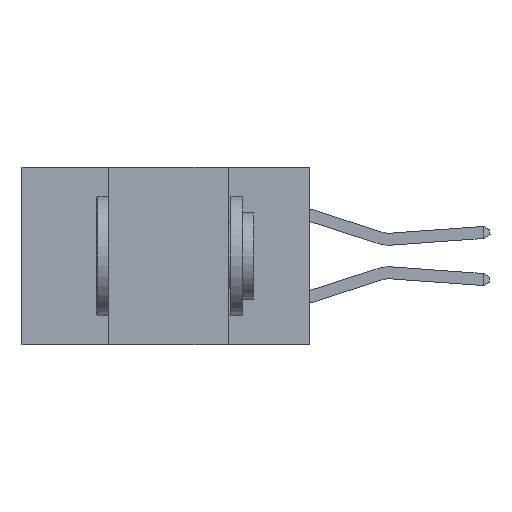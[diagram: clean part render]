
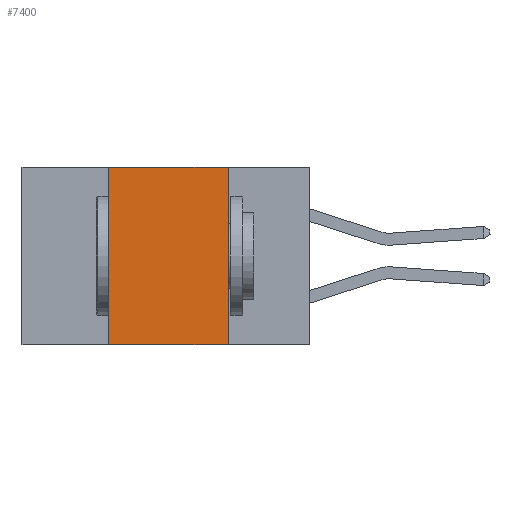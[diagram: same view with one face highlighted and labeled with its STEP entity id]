
A CAD part, left-side view. The second image highlights one B-rep face of the part: STEP entity #7400.
In plain terms, the highlighted planar face has unit normal (-1, 0, 0).
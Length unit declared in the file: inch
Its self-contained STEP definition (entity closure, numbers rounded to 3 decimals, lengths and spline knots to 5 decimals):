
#348 = DIRECTION ( 'NONE',  ( 1., 0., 0. ) ) ;
#670 = DIRECTION ( 'NONE',  ( 0., -1., 0. ) ) ;
#845 = CARTESIAN_POINT ( 'NONE',  ( 0., 0.6, 0. ) ) ;
#970 = VERTEX_POINT ( 'NONE', #16342 ) ;
#4624 = LINE ( 'NONE', #15076, #7123 ) ;
#5037 = EDGE_CURVE ( 'NONE', #16337, #5804, #14171, .T. ) ;
#5453 = ORIENTED_EDGE ( 'NONE', *, *, #18565, .T. ) ;
#5486 = VECTOR ( 'NONE', #18197, 39.37008 ) ;
#5804 = VERTEX_POINT ( 'NONE', #15506 ) ;
#5982 = ORIENTED_EDGE ( 'NONE', *, *, #14005, .F. ) ;
#6254 = EDGE_LOOP ( 'NONE', ( #5982, #7475, #9802, #5453 ) ) ;
#6794 = LINE ( 'NONE', #16508, #7512 ) ;
#7123 = VECTOR ( 'NONE', #11762, 39.37008 ) ;
#7400 = ADVANCED_FACE ( 'NONE', ( #11366 ), #9693, .F. ) ;
#7475 = ORIENTED_EDGE ( 'NONE', *, *, #5037, .F. ) ;
#7512 = VECTOR ( 'NONE', #670, 39.37008 ) ;
#7846 = AXIS2_PLACEMENT_3D ( 'NONE', #16038, #348, #16376 ) ;
#7856 = CARTESIAN_POINT ( 'NONE',  ( 0., 0.42, -0.37 ) ) ;
#8217 = DIRECTION ( 'NONE',  ( 0., 0., -1. ) ) ;
#8296 = EDGE_CURVE ( 'NONE', #15723, #16337, #4624, .T. ) ;
#9693 = PLANE ( 'NONE',  #7846 ) ;
#9802 = ORIENTED_EDGE ( 'NONE', *, *, #8296, .F. ) ;
#10439 = CARTESIAN_POINT ( 'NONE',  ( 0., 0.42, 0. ) ) ;
#11366 = FACE_OUTER_BOUND ( 'NONE', #6254, .T. ) ;
#11762 = DIRECTION ( 'NONE',  ( 0., 0., 1. ) ) ;
#12466 = LINE ( 'NONE', #17686, #19865 ) ;
#14005 = EDGE_CURVE ( 'NONE', #5804, #970, #12466, .T. ) ;
#14171 = LINE ( 'NONE', #845, #5486 ) ;
#15076 = CARTESIAN_POINT ( 'NONE',  ( 0., 0.42, 0. ) ) ;
#15506 = CARTESIAN_POINT ( 'NONE',  ( 0., 0.17, 0. ) ) ;
#15723 = VERTEX_POINT ( 'NONE', #7856 ) ;
#16038 = CARTESIAN_POINT ( 'NONE',  ( 0., 0.6, 0. ) ) ;
#16337 = VERTEX_POINT ( 'NONE', #10439 ) ;
#16342 = CARTESIAN_POINT ( 'NONE',  ( 0., 0.17, -0.37 ) ) ;
#16376 = DIRECTION ( 'NONE',  ( 0., 0., -1. ) ) ;
#16508 = CARTESIAN_POINT ( 'NONE',  ( 0., 0.6, -0.37 ) ) ;
#17686 = CARTESIAN_POINT ( 'NONE',  ( 0., 0.17, 0. ) ) ;
#18197 = DIRECTION ( 'NONE',  ( 0., -1., 0. ) ) ;
#18565 = EDGE_CURVE ( 'NONE', #15723, #970, #6794, .T. ) ;
#19865 = VECTOR ( 'NONE', #8217, 39.37008 ) ;
